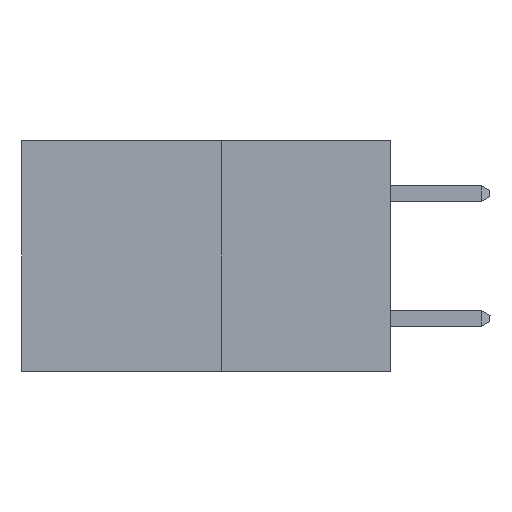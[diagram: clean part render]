
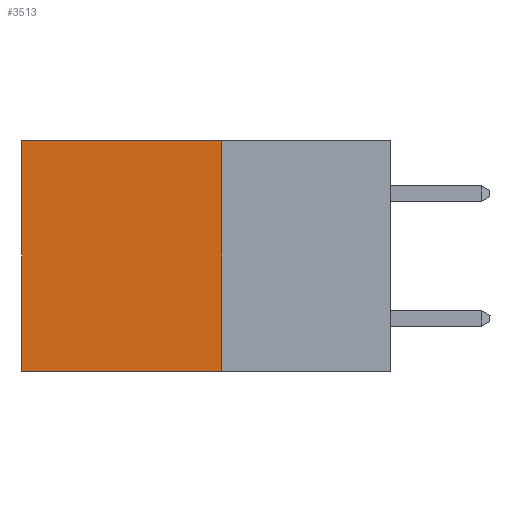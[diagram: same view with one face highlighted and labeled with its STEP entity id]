
A CAD part, left-side view. The second image highlights one B-rep face of the part: STEP entity #3513.
In plain terms, the highlighted planar face has unit normal (-1, 0, 0).
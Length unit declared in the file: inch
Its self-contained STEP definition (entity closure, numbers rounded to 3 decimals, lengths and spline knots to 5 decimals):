
#11 = CARTESIAN_POINT ( 'NONE',  ( 0.277, 0.59, 0. ) ) ;
#57 = CARTESIAN_POINT ( 'NONE',  ( 0.277, 0.27, -0.37 ) ) ;
#154 = DIRECTION ( 'NONE',  ( 0., 1., 0. ) ) ;
#266 = DIRECTION ( 'NONE',  ( 0., 1., 0. ) ) ;
#655 = DIRECTION ( 'NONE',  ( 0., 0., -1. ) ) ;
#815 = LINE ( 'NONE', #6875, #1490 ) ;
#909 = VERTEX_POINT ( 'NONE', #10368 ) ;
#1074 = CARTESIAN_POINT ( 'NONE',  ( 0.277, 0.27, -0.37 ) ) ;
#1224 = EDGE_CURVE ( 'NONE', #1798, #10124, #6216, .T. ) ;
#1406 = ORIENTED_EDGE ( 'NONE', *, *, #1776, .F. ) ;
#1490 = VECTOR ( 'NONE', #655, 39.37008 ) ;
#1776 = EDGE_CURVE ( 'NONE', #909, #1798, #5528, .T. ) ;
#1798 = VERTEX_POINT ( 'NONE', #57 ) ;
#2208 = AXIS2_PLACEMENT_3D ( 'NONE', #4945, #5142, #5049 ) ;
#2393 = DIRECTION ( 'NONE',  ( 0., 0., -1. ) ) ;
#2832 = CARTESIAN_POINT ( 'NONE',  ( 0.277, 0.27, -0.37 ) ) ;
#2946 = FACE_OUTER_BOUND ( 'NONE', #8863, .T. ) ;
#3045 = LINE ( 'NONE', #4054, #5006 ) ;
#3513 = ADVANCED_FACE ( 'NONE', ( #2946 ), #4813, .F. ) ;
#4054 = CARTESIAN_POINT ( 'NONE',  ( 0.277, 0.27, 0. ) ) ;
#4813 = PLANE ( 'NONE',  #2208 ) ;
#4945 = CARTESIAN_POINT ( 'NONE',  ( 0.277, 0.27, -0.37 ) ) ;
#5006 = VECTOR ( 'NONE', #154, 39.37008 ) ;
#5049 = DIRECTION ( 'NONE',  ( 0., 0., -1. ) ) ;
#5142 = DIRECTION ( 'NONE',  ( 1., 0., 0. ) ) ;
#5528 = LINE ( 'NONE', #2832, #9153 ) ;
#6119 = ORIENTED_EDGE ( 'NONE', *, *, #8806, .T. ) ;
#6216 = LINE ( 'NONE', #1074, #9667 ) ;
#6875 = CARTESIAN_POINT ( 'NONE',  ( 0.277, 0.59, -0.37 ) ) ;
#7873 = ORIENTED_EDGE ( 'NONE', *, *, #8062, .T. ) ;
#8062 = EDGE_CURVE ( 'NONE', #9974, #10124, #815, .T. ) ;
#8806 = EDGE_CURVE ( 'NONE', #909, #9974, #3045, .T. ) ;
#8863 = EDGE_LOOP ( 'NONE', ( #7873, #9596, #1406, #6119 ) ) ;
#9153 = VECTOR ( 'NONE', #2393, 39.37008 ) ;
#9596 = ORIENTED_EDGE ( 'NONE', *, *, #1224, .F. ) ;
#9667 = VECTOR ( 'NONE', #266, 39.37008 ) ;
#9974 = VERTEX_POINT ( 'NONE', #11 ) ;
#10069 = CARTESIAN_POINT ( 'NONE',  ( 0.277, 0.59, -0.37 ) ) ;
#10124 = VERTEX_POINT ( 'NONE', #10069 ) ;
#10368 = CARTESIAN_POINT ( 'NONE',  ( 0.277, 0.27, 0. ) ) ;
